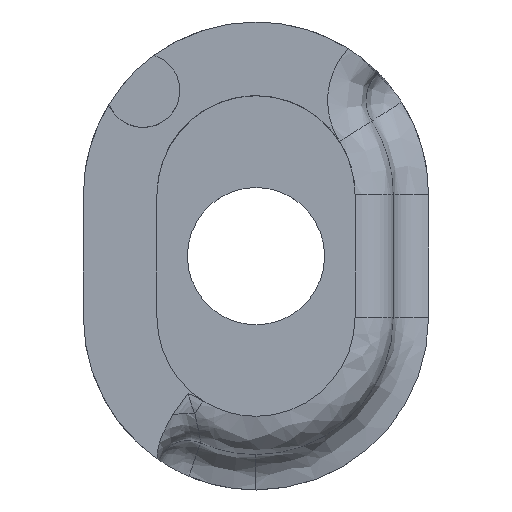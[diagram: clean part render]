
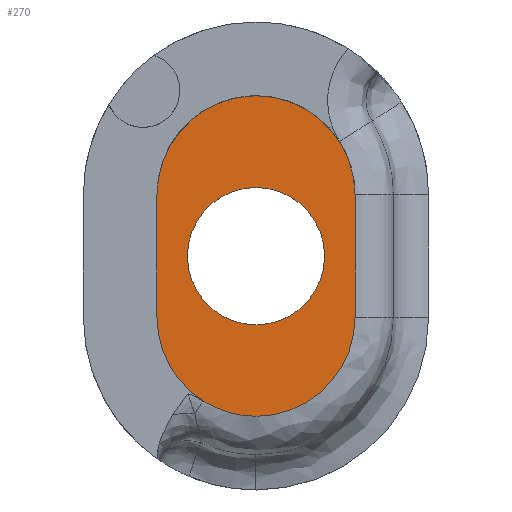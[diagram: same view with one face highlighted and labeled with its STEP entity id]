
A CAD part, top view. The second image highlights one B-rep face of the part: STEP entity #270.
In plain terms, the highlighted planar face has unit normal (0, 0, 1).
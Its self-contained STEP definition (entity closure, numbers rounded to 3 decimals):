
#64 = CARTESIAN_POINT ( 'NONE',  ( 19.216, 59.227, 155.898 ) ) ;
#93 = DIRECTION ( 'NONE',  ( 0., 1., 0. ) ) ;
#101 = CARTESIAN_POINT ( 'NONE',  ( 23.255, 59.227, 155.898 ) ) ;
#114 = VERTEX_POINT ( 'NONE', #64 ) ;
#148 = CARTESIAN_POINT ( 'NONE',  ( 27.294, 54.223, 155.898 ) ) ;
#158 = CARTESIAN_POINT ( 'NONE',  ( 27.294, 59.227, 155.898 ) ) ;
#211 = CARTESIAN_POINT ( 'NONE',  ( 23.255, 59.525, 155.898 ) ) ;
#270 = ADVANCED_FACE ( 'NONE', ( #808, #837 ), #991, .F. ) ;
#366 = VERTEX_POINT ( 'NONE', #148 ) ;
#409 = CARTESIAN_POINT ( 'NONE',  ( 23.255, 50.184, 155.898 ) ) ;
#414 = CARTESIAN_POINT ( 'NONE',  ( 23.255, 53.925, 155.898 ) ) ;
#461 = VECTOR ( 'NONE', #947, 1000. ) ;
#464 = LINE ( 'NONE', #1151, #461 ) ;
#489 = CIRCLE ( 'NONE', #611, 4.039 ) ;
#494 = VECTOR ( 'NONE', #93, 1000. ) ;
#496 = LINE ( 'NONE', #1706, #494 ) ;
#497 = CIRCLE ( 'NONE', #607, 2.8 ) ;
#516 = CIRCLE ( 'NONE', #620, 4.039 ) ;
#596 = CIRCLE ( 'NONE', #659, 2.8 ) ;
#607 = AXIS2_PLACEMENT_3D ( 'NONE', #1141, #1144, #1149 ) ;
#611 = AXIS2_PLACEMENT_3D ( 'NONE', #1133, #1059, #1064 ) ;
#620 = AXIS2_PLACEMENT_3D ( 'NONE', #1089, #1137, #1112 ) ;
#651 = CIRCLE ( 'NONE', #687, 4.039 ) ;
#659 = AXIS2_PLACEMENT_3D ( 'NONE', #1405, #1371, #1375 ) ;
#687 = AXIS2_PLACEMENT_3D ( 'NONE', #1200, #1197, #1598 ) ;
#734 = ORIENTED_EDGE ( 'NONE', *, *, #961, .T. ) ;
#758 = DIRECTION ( 'NONE',  ( 0., 1., 0. ) ) ;
#778 = AXIS2_PLACEMENT_3D ( 'NONE', #101, #1404, #758 ) ;
#808 = FACE_BOUND ( 'NONE', #971, .T. ) ;
#822 = VERTEX_POINT ( 'NONE', #834 ) ;
#834 = CARTESIAN_POINT ( 'NONE',  ( 19.216, 54.223, 155.898 ) ) ;
#837 = FACE_OUTER_BOUND ( 'NONE', #1213, .T. ) ;
#940 = ORIENTED_EDGE ( 'NONE', *, *, #1101, .T. ) ;
#947 = DIRECTION ( 'NONE',  ( 0., -1., 0. ) ) ;
#961 = EDGE_CURVE ( 'NONE', #1289, #366, #651, .T. ) ;
#971 = EDGE_LOOP ( 'NONE', ( #1093, #1523 ) ) ;
#990 = EDGE_CURVE ( 'NONE', #1560, #1255, #596, .T. ) ;
#991 = PLANE ( 'NONE',  #778 ) ;
#1001 = ORIENTED_EDGE ( 'NONE', *, *, #1067, .T. ) ;
#1035 = ORIENTED_EDGE ( 'NONE', *, *, #1091, .T. ) ;
#1059 = DIRECTION ( 'NONE',  ( 0., 0., 1. ) ) ;
#1064 = DIRECTION ( 'NONE',  ( 0., 1., 0. ) ) ;
#1067 = EDGE_CURVE ( 'NONE', #822, #1289, #516, .T. ) ;
#1081 = EDGE_CURVE ( 'NONE', #366, #1677, #496, .T. ) ;
#1089 = CARTESIAN_POINT ( 'NONE',  ( 23.255, 54.223, 155.898 ) ) ;
#1091 = EDGE_CURVE ( 'NONE', #1677, #114, #489, .T. ) ;
#1093 = ORIENTED_EDGE ( 'NONE', *, *, #1095, .F. ) ;
#1094 = ORIENTED_EDGE ( 'NONE', *, *, #1081, .T. ) ;
#1095 = EDGE_CURVE ( 'NONE', #1255, #1560, #497, .T. ) ;
#1101 = EDGE_CURVE ( 'NONE', #114, #822, #464, .T. ) ;
#1112 = DIRECTION ( 'NONE',  ( 0., 1., 0. ) ) ;
#1133 = CARTESIAN_POINT ( 'NONE',  ( 23.255, 59.227, 155.898 ) ) ;
#1137 = DIRECTION ( 'NONE',  ( 0., 0., 1. ) ) ;
#1141 = CARTESIAN_POINT ( 'NONE',  ( 23.255, 56.725, 155.898 ) ) ;
#1144 = DIRECTION ( 'NONE',  ( 0., 0., 1. ) ) ;
#1149 = DIRECTION ( 'NONE',  ( 0., -1., 0. ) ) ;
#1151 = CARTESIAN_POINT ( 'NONE',  ( 19.216, 59.227, 155.898 ) ) ;
#1197 = DIRECTION ( 'NONE',  ( 0., 0., 1. ) ) ;
#1200 = CARTESIAN_POINT ( 'NONE',  ( 23.255, 54.223, 155.898 ) ) ;
#1213 = EDGE_LOOP ( 'NONE', ( #1035, #940, #1001, #734, #1094 ) ) ;
#1255 = VERTEX_POINT ( 'NONE', #414 ) ;
#1289 = VERTEX_POINT ( 'NONE', #409 ) ;
#1371 = DIRECTION ( 'NONE',  ( 0., 0., 1. ) ) ;
#1375 = DIRECTION ( 'NONE',  ( 0., -1., 0. ) ) ;
#1404 = DIRECTION ( 'NONE',  ( 0., 0., -1. ) ) ;
#1405 = CARTESIAN_POINT ( 'NONE',  ( 23.255, 56.725, 155.898 ) ) ;
#1523 = ORIENTED_EDGE ( 'NONE', *, *, #990, .F. ) ;
#1560 = VERTEX_POINT ( 'NONE', #211 ) ;
#1598 = DIRECTION ( 'NONE',  ( 0., 1., 0. ) ) ;
#1677 = VERTEX_POINT ( 'NONE', #158 ) ;
#1706 = CARTESIAN_POINT ( 'NONE',  ( 27.294, 54.223, 155.898 ) ) ;
